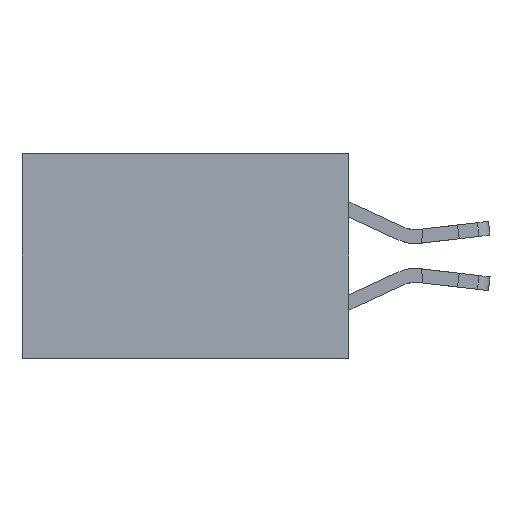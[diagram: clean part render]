
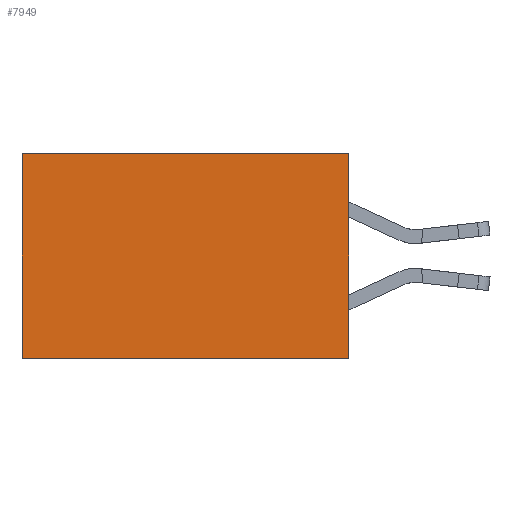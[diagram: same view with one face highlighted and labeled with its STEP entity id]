
A CAD part, left-side view. The second image highlights one B-rep face of the part: STEP entity #7949.
In plain terms, the highlighted planar face has unit normal (-1, 0, 0).
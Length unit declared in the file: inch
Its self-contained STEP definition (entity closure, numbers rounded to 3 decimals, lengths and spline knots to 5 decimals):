
#1339 = VERTEX_POINT ( 'NONE', #7107 ) ;
#1760 = AXIS2_PLACEMENT_3D ( 'NONE', #4636, #4522, #4518 ) ;
#2053 = FACE_OUTER_BOUND ( 'NONE', #18778, .T. ) ;
#2449 = CARTESIAN_POINT ( 'NONE',  ( 0.277, 0., 0. ) ) ;
#3132 = ORIENTED_EDGE ( 'NONE', *, *, #14969, .T. ) ;
#3139 = VECTOR ( 'NONE', #17796, 39.37008 ) ;
#3568 = VERTEX_POINT ( 'NONE', #19020 ) ;
#4150 = DIRECTION ( 'NONE',  ( 0., 0., -1. ) ) ;
#4491 = CARTESIAN_POINT ( 'NONE',  ( 0.277, 0.59, -0.37 ) ) ;
#4518 = DIRECTION ( 'NONE',  ( 0., 0., -1. ) ) ;
#4522 = DIRECTION ( 'NONE',  ( 1., 0., 0. ) ) ;
#4563 = PLANE ( 'NONE',  #1760 ) ;
#4636 = CARTESIAN_POINT ( 'NONE',  ( 0.277, 0., -0.37 ) ) ;
#6514 = ORIENTED_EDGE ( 'NONE', *, *, #9357, .T. ) ;
#6765 = EDGE_CURVE ( 'NONE', #17398, #3568, #10987, .T. ) ;
#7107 = CARTESIAN_POINT ( 'NONE',  ( 0.277, 0.59, 0. ) ) ;
#7949 = ADVANCED_FACE ( 'NONE', ( #2053 ), #4563, .F. ) ;
#8793 = VECTOR ( 'NONE', #4150, 39.37008 ) ;
#9357 = EDGE_CURVE ( 'NONE', #1339, #16398, #12825, .T. ) ;
#9769 = CARTESIAN_POINT ( 'NONE',  ( 0.277, 0., -0.37 ) ) ;
#10987 = LINE ( 'NONE', #9769, #14560 ) ;
#11053 = ORIENTED_EDGE ( 'NONE', *, *, #18959, .F. ) ;
#12825 = LINE ( 'NONE', #4491, #8793 ) ;
#13185 = DIRECTION ( 'NONE',  ( 0., 1., 0. ) ) ;
#14102 = VECTOR ( 'NONE', #13185, 39.37008 ) ;
#14560 = VECTOR ( 'NONE', #17267, 39.37008 ) ;
#14739 = CARTESIAN_POINT ( 'NONE',  ( 0.277, 0., 0. ) ) ;
#14756 = CARTESIAN_POINT ( 'NONE',  ( 0.277, 0., -0.37 ) ) ;
#14969 = EDGE_CURVE ( 'NONE', #17398, #1339, #15067, .T. ) ;
#15067 = LINE ( 'NONE', #14739, #14102 ) ;
#15640 = CARTESIAN_POINT ( 'NONE',  ( 0.277, 0.59, -0.37 ) ) ;
#16398 = VERTEX_POINT ( 'NONE', #15640 ) ;
#17267 = DIRECTION ( 'NONE',  ( 0., 0., -1. ) ) ;
#17398 = VERTEX_POINT ( 'NONE', #2449 ) ;
#17796 = DIRECTION ( 'NONE',  ( 0., 1., 0. ) ) ;
#17956 = ORIENTED_EDGE ( 'NONE', *, *, #6765, .F. ) ;
#18778 = EDGE_LOOP ( 'NONE', ( #6514, #11053, #17956, #3132 ) ) ;
#18876 = LINE ( 'NONE', #14756, #3139 ) ;
#18959 = EDGE_CURVE ( 'NONE', #3568, #16398, #18876, .T. ) ;
#19020 = CARTESIAN_POINT ( 'NONE',  ( 0.277, 0., -0.37 ) ) ;
